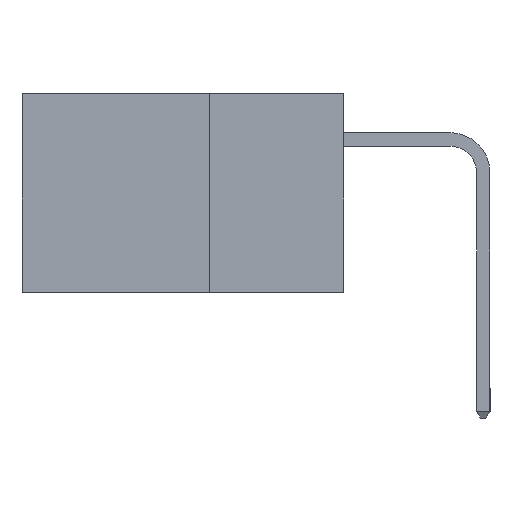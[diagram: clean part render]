
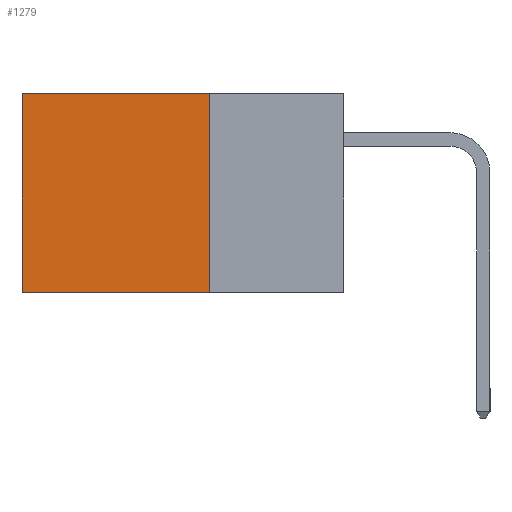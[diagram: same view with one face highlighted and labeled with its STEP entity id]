
A CAD part, left-side view. The second image highlights one B-rep face of the part: STEP entity #1279.
In plain terms, the highlighted planar face has unit normal (-1, 0, 0).
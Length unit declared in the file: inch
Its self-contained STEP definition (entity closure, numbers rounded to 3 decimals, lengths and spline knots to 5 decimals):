
#391 = DIRECTION ( 'NONE',  ( 0., 1., 0. ) ) ;
#462 = LINE ( 'NONE', #13588, #2292 ) ;
#798 = LINE ( 'NONE', #13703, #5341 ) ;
#1279 = ADVANCED_FACE ( 'NONE', ( #22545 ), #19823, .F. ) ;
#2230 = DIRECTION ( 'NONE',  ( 0., 0., -1. ) ) ;
#2292 = VECTOR ( 'NONE', #2230, 39.37008 ) ;
#3000 = VERTEX_POINT ( 'NONE', #18845 ) ;
#3122 = ORIENTED_EDGE ( 'NONE', *, *, #22679, .T. ) ;
#3818 = EDGE_CURVE ( 'NONE', #12616, #20703, #798, .T. ) ;
#4183 = VERTEX_POINT ( 'NONE', #12777 ) ;
#4484 = EDGE_CURVE ( 'NONE', #3000, #20703, #462, .T. ) ;
#5341 = VECTOR ( 'NONE', #391, 39.37008 ) ;
#10035 = DIRECTION ( 'NONE',  ( 0., 0., -1. ) ) ;
#10274 = VECTOR ( 'NONE', #10035, 39.37008 ) ;
#10542 = DIRECTION ( 'NONE',  ( 0., 1., 0. ) ) ;
#10884 = LINE ( 'NONE', #21406, #10274 ) ;
#12454 = CARTESIAN_POINT ( 'NONE',  ( 0.298, 0.6, -0.37 ) ) ;
#12616 = VERTEX_POINT ( 'NONE', #12702 ) ;
#12702 = CARTESIAN_POINT ( 'NONE',  ( 0.298, 0.25, -0.37 ) ) ;
#12777 = CARTESIAN_POINT ( 'NONE',  ( 0.298, 0.25, 0. ) ) ;
#13442 = ORIENTED_EDGE ( 'NONE', *, *, #3818, .F. ) ;
#13588 = CARTESIAN_POINT ( 'NONE',  ( 0.298, 0.6, 0. ) ) ;
#13703 = CARTESIAN_POINT ( 'NONE',  ( 0.298, 0.25, -0.37 ) ) ;
#14558 = DIRECTION ( 'NONE',  ( 0., 0., -1. ) ) ;
#14581 = DIRECTION ( 'NONE',  ( 1., 0., 0. ) ) ;
#15238 = EDGE_LOOP ( 'NONE', ( #19555, #13442, #17053, #3122 ) ) ;
#15285 = AXIS2_PLACEMENT_3D ( 'NONE', #19502, #14581, #14558 ) ;
#17053 = ORIENTED_EDGE ( 'NONE', *, *, #19539, .F. ) ;
#18736 = VECTOR ( 'NONE', #10542, 39.37008 ) ;
#18845 = CARTESIAN_POINT ( 'NONE',  ( 0.298, 0.6, 0. ) ) ;
#19329 = LINE ( 'NONE', #23701, #18736 ) ;
#19502 = CARTESIAN_POINT ( 'NONE',  ( 0.298, 0.25, 0. ) ) ;
#19539 = EDGE_CURVE ( 'NONE', #4183, #12616, #10884, .T. ) ;
#19555 = ORIENTED_EDGE ( 'NONE', *, *, #4484, .T. ) ;
#19823 = PLANE ( 'NONE',  #15285 ) ;
#20703 = VERTEX_POINT ( 'NONE', #12454 ) ;
#21406 = CARTESIAN_POINT ( 'NONE',  ( 0.298, 0.25, 0. ) ) ;
#22545 = FACE_OUTER_BOUND ( 'NONE', #15238, .T. ) ;
#22679 = EDGE_CURVE ( 'NONE', #4183, #3000, #19329, .T. ) ;
#23701 = CARTESIAN_POINT ( 'NONE',  ( 0.298, 0.25, 0. ) ) ;
